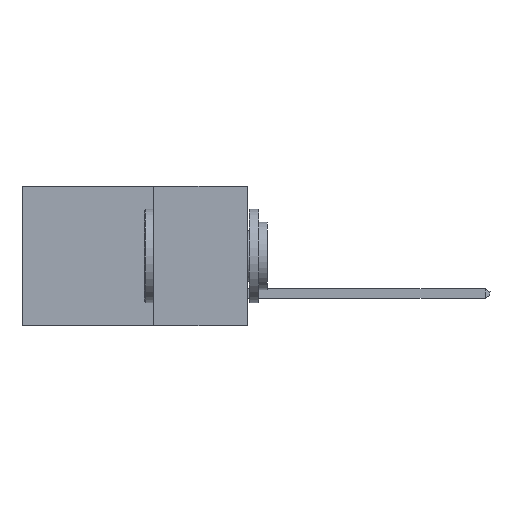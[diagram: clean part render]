
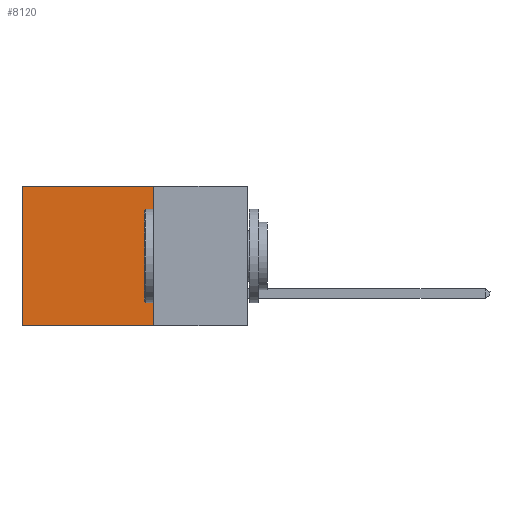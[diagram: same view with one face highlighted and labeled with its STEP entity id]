
A CAD part, left-side view. The second image highlights one B-rep face of the part: STEP entity #8120.
In plain terms, the highlighted planar face has unit normal (-1, 0, 0).
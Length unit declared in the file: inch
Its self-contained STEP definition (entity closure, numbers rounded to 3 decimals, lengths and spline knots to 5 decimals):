
#334 = VERTEX_POINT ( 'NONE', #2270 ) ;
#523 = LINE ( 'NONE', #2821, #4863 ) ;
#572 = DIRECTION ( 'NONE',  ( 0., 0., -1. ) ) ;
#1011 = VECTOR ( 'NONE', #6316, 39.37008 ) ;
#1302 = DIRECTION ( 'NONE',  ( 0., 1., 0. ) ) ;
#1479 = DIRECTION ( 'NONE',  ( 0., 0., -1. ) ) ;
#1754 = VERTEX_POINT ( 'NONE', #3055 ) ;
#2073 = LINE ( 'NONE', #3606, #8229 ) ;
#2270 = CARTESIAN_POINT ( 'NONE',  ( 0.2615, 0.25, -0.37 ) ) ;
#2299 = CARTESIAN_POINT ( 'NONE',  ( 0.2615, 0.25, -0.37 ) ) ;
#2680 = VERTEX_POINT ( 'NONE', #3488 ) ;
#2821 = CARTESIAN_POINT ( 'NONE',  ( 0.2615, 0.25, -0.37 ) ) ;
#2977 = ORIENTED_EDGE ( 'NONE', *, *, #3424, .F. ) ;
#3055 = CARTESIAN_POINT ( 'NONE',  ( 0.2615, 0.6, -0.37 ) ) ;
#3424 = EDGE_CURVE ( 'NONE', #334, #1754, #9459, .T. ) ;
#3488 = CARTESIAN_POINT ( 'NONE',  ( 0.2615, 0.25, 0. ) ) ;
#3606 = CARTESIAN_POINT ( 'NONE',  ( 0.2615, 0.6, -0.37 ) ) ;
#3813 = EDGE_CURVE ( 'NONE', #2680, #8216, #5566, .T. ) ;
#3857 = EDGE_CURVE ( 'NONE', #2680, #334, #523, .T. ) ;
#4239 = EDGE_LOOP ( 'NONE', ( #5133, #2977, #5997, #6174 ) ) ;
#4608 = PLANE ( 'NONE',  #8862 ) ;
#4863 = VECTOR ( 'NONE', #572, 39.37008 ) ;
#5133 = ORIENTED_EDGE ( 'NONE', *, *, #7215, .T. ) ;
#5566 = LINE ( 'NONE', #8501, #1011 ) ;
#5769 = DIRECTION ( 'NONE',  ( 0., 0., -1. ) ) ;
#5997 = ORIENTED_EDGE ( 'NONE', *, *, #3857, .F. ) ;
#6174 = ORIENTED_EDGE ( 'NONE', *, *, #3813, .T. ) ;
#6316 = DIRECTION ( 'NONE',  ( 0., 1., 0. ) ) ;
#7215 = EDGE_CURVE ( 'NONE', #8216, #1754, #2073, .T. ) ;
#7924 = CARTESIAN_POINT ( 'NONE',  ( 0.2615, 0.25, -0.37 ) ) ;
#8120 = ADVANCED_FACE ( 'NONE', ( #8252 ), #4608, .F. ) ;
#8201 = DIRECTION ( 'NONE',  ( 1., 0., 0. ) ) ;
#8216 = VERTEX_POINT ( 'NONE', #8836 ) ;
#8229 = VECTOR ( 'NONE', #5769, 39.37008 ) ;
#8252 = FACE_OUTER_BOUND ( 'NONE', #4239, .T. ) ;
#8501 = CARTESIAN_POINT ( 'NONE',  ( 0.2615, 0.25, 0. ) ) ;
#8836 = CARTESIAN_POINT ( 'NONE',  ( 0.2615, 0.6, 0. ) ) ;
#8862 = AXIS2_PLACEMENT_3D ( 'NONE', #2299, #8201, #1479 ) ;
#9132 = VECTOR ( 'NONE', #1302, 39.37008 ) ;
#9459 = LINE ( 'NONE', #7924, #9132 ) ;
